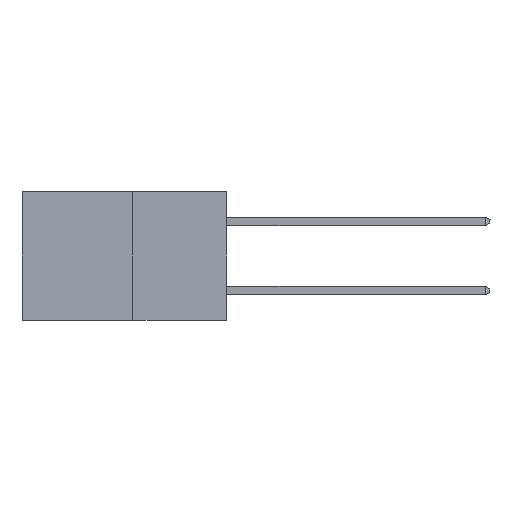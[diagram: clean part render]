
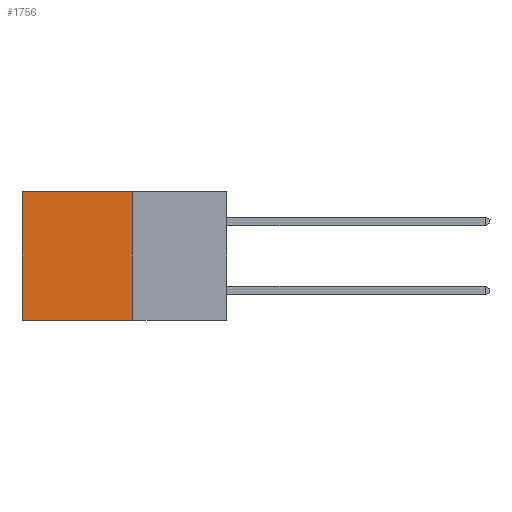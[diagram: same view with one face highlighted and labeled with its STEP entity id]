
A CAD part, left-side view. The second image highlights one B-rep face of the part: STEP entity #1756.
In plain terms, the highlighted planar face has unit normal (-1, 0, 0).
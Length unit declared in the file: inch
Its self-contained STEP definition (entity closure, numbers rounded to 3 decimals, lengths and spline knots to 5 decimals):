
#59 = LINE ( 'NONE', #3670, #8965 ) ;
#121 = DIRECTION ( 'NONE',  ( 0., 0., -1. ) ) ;
#313 = FACE_OUTER_BOUND ( 'NONE', #10400, .T. ) ;
#417 = ORIENTED_EDGE ( 'NONE', *, *, #10064, .T. ) ;
#525 = EDGE_CURVE ( 'NONE', #9411, #7521, #1856, .T. ) ;
#738 = VECTOR ( 'NONE', #5758, 39.37008 ) ;
#1022 = DIRECTION ( 'NONE',  ( 0., 0., -1. ) ) ;
#1756 = ADVANCED_FACE ( 'NONE', ( #313 ), #7662, .F. ) ;
#1856 = LINE ( 'NONE', #5840, #10555 ) ;
#2206 = CARTESIAN_POINT ( 'NONE',  ( 0.277, 0.27, -0.37 ) ) ;
#2301 = CARTESIAN_POINT ( 'NONE',  ( 0.277, 0.59, -0.37 ) ) ;
#2551 = LINE ( 'NONE', #2206, #738 ) ;
#2914 = VERTEX_POINT ( 'NONE', #3486 ) ;
#3486 = CARTESIAN_POINT ( 'NONE',  ( 0.277, 0.27, -0.37 ) ) ;
#3670 = CARTESIAN_POINT ( 'NONE',  ( 0.277, 0.27, -0.37 ) ) ;
#4147 = DIRECTION ( 'NONE',  ( 0., 0., -1. ) ) ;
#4170 = CARTESIAN_POINT ( 'NONE',  ( 0.277, 0.27, 0. ) ) ;
#5758 = DIRECTION ( 'NONE',  ( 0., 1., 0. ) ) ;
#5840 = CARTESIAN_POINT ( 'NONE',  ( 0.277, 0.59, -0.37 ) ) ;
#6437 = CARTESIAN_POINT ( 'NONE',  ( 0.277, 0.27, 0. ) ) ;
#6483 = EDGE_CURVE ( 'NONE', #8466, #2914, #59, .T. ) ;
#6724 = EDGE_CURVE ( 'NONE', #2914, #7521, #2551, .T. ) ;
#6929 = CARTESIAN_POINT ( 'NONE',  ( 0.277, 0.27, -0.37 ) ) ;
#7506 = ORIENTED_EDGE ( 'NONE', *, *, #6724, .F. ) ;
#7521 = VERTEX_POINT ( 'NONE', #2301 ) ;
#7553 = LINE ( 'NONE', #4170, #9387 ) ;
#7655 = CARTESIAN_POINT ( 'NONE',  ( 0.277, 0.59, 0. ) ) ;
#7662 = PLANE ( 'NONE',  #10874 ) ;
#8466 = VERTEX_POINT ( 'NONE', #6437 ) ;
#8493 = DIRECTION ( 'NONE',  ( 1., 0., 0. ) ) ;
#8965 = VECTOR ( 'NONE', #121, 39.37008 ) ;
#9160 = DIRECTION ( 'NONE',  ( 0., 1., 0. ) ) ;
#9230 = ORIENTED_EDGE ( 'NONE', *, *, #6483, .F. ) ;
#9387 = VECTOR ( 'NONE', #9160, 39.37008 ) ;
#9411 = VERTEX_POINT ( 'NONE', #7655 ) ;
#9734 = ORIENTED_EDGE ( 'NONE', *, *, #525, .T. ) ;
#10064 = EDGE_CURVE ( 'NONE', #8466, #9411, #7553, .T. ) ;
#10400 = EDGE_LOOP ( 'NONE', ( #9734, #7506, #9230, #417 ) ) ;
#10555 = VECTOR ( 'NONE', #1022, 39.37008 ) ;
#10874 = AXIS2_PLACEMENT_3D ( 'NONE', #6929, #8493, #4147 ) ;
